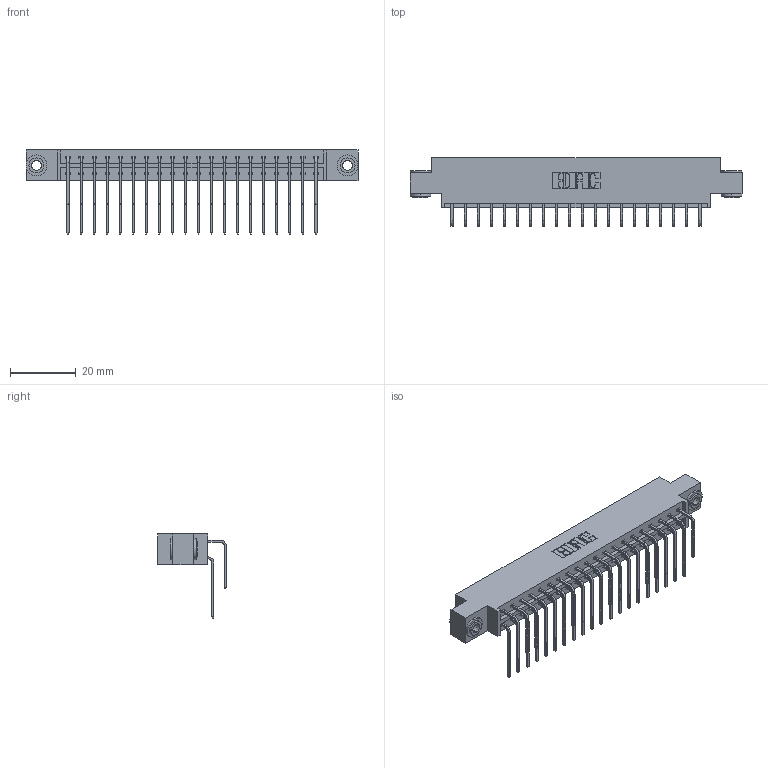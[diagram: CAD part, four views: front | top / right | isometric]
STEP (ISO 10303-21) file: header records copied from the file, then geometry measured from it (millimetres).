
FILE_DESCRIPTION (( 'STEP AP203' ), '1' );
FILE_NAME ('333-040-559-803.STEP', '2018-08-03T14:56:28', ( '' ), ( '' ), 'SwSTEP 2.0', 'SolidWorks 2016', '' );
FILE_SCHEMA (( 'CONFIG_CONTROL_DESIGN' ));
Length unit declared in the file: inch
Products named in the file (5): 333-040-559-803; 333 Part_Offset - .156 Dia - TH; 345-292-001_558 559 Tail - 1; 345-292-001_559 Tail - 2; 345-250-002_345-250-002-102
Assembly tree (43 placements, depth 2):
  333-040-559-803
    333 Part_Offset - .156 Dia - TH
    345-292-001_558 559 Tail - 1  x20
    345-292-001_559 Tail - 2  x20
    345-250-002_345-250-002-102  x2
Bounding box: 100.79 x 20.9 x 25.53 mm (x, y, z)
Volume: 10106.4 mm3; surface area: 13303 mm2
Topology: 43 solids, 43 shells, 2316 faces, 6839 edges, 4502 vertices
Faces by surface type: plane 1604, cylinder 704, cone 8
Entity records: 18278 total; most frequent: CARTESIAN_POINT 3084, ORIENTED_EDGE 2962, DIRECTION 2687, EDGE_CURVE 1481, VECTOR 1289, LINE 1289, VERTEX_POINT 982, AXIS2_PLACEMENT_3D 699
